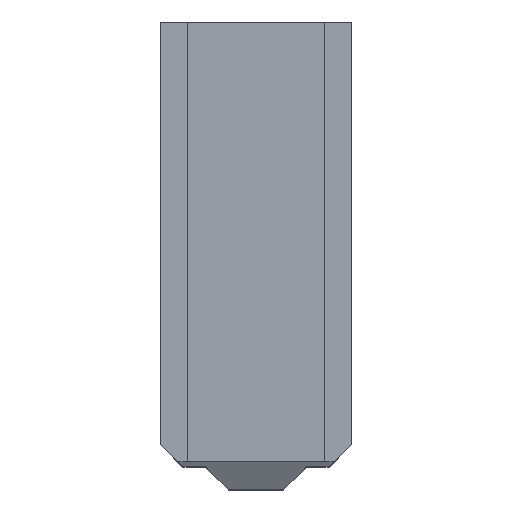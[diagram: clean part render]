
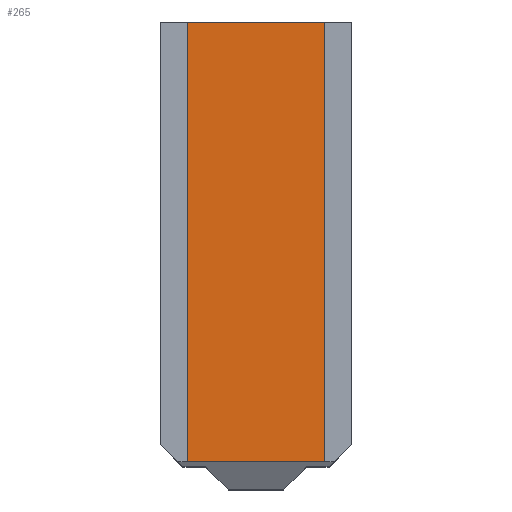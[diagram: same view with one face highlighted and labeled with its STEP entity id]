
A CAD part, top view. The second image highlights one B-rep face of the part: STEP entity #265.
In plain terms, the highlighted planar face has unit normal (0, 0, 1).
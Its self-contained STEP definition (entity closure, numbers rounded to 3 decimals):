
#164 = VERTEX_POINT ( 'NONE', #906 ) ;
#171 = VERTEX_POINT ( 'NONE', #882 ) ;
#204 = EDGE_LOOP ( 'NONE', ( #1276, #1154, #1141, #1271 ) ) ;
#229 = EDGE_CURVE ( 'NONE', #801, #812, #964, .T. ) ;
#265 = ADVANCED_FACE ( 'NONE', ( #513 ), #1112, .T. ) ;
#314 = EDGE_CURVE ( 'NONE', #171, #801, #1426, .T. ) ;
#315 = EDGE_CURVE ( 'NONE', #164, #171, #1428, .T. ) ;
#341 = EDGE_CURVE ( 'NONE', #812, #164, #1507, .T. ) ;
#444 = VECTOR ( 'NONE', #944, 1000. ) ;
#513 = FACE_OUTER_BOUND ( 'NONE', #204, .T. ) ;
#526 = AXIS2_PLACEMENT_3D ( 'NONE', #1099, #1109, #1105 ) ;
#599 = VECTOR ( 'NONE', #1427, 1000. ) ;
#608 = VECTOR ( 'NONE', #1468, 1000. ) ;
#624 = VECTOR ( 'NONE', #1511, 1000. ) ;
#801 = VERTEX_POINT ( 'NONE', #1573 ) ;
#812 = VERTEX_POINT ( 'NONE', #1560 ) ;
#882 = CARTESIAN_POINT ( 'NONE',  ( 15.128, -20.109, 114.412 ) ) ;
#906 = CARTESIAN_POINT ( 'NONE',  ( -15.113, -20.109, 114.412 ) ) ;
#943 = CARTESIAN_POINT ( 'NONE',  ( 0., 76.858, 114.412 ) ) ;
#944 = DIRECTION ( 'NONE',  ( -1., 0., 0. ) ) ;
#964 = LINE ( 'NONE', #943, #444 ) ;
#1099 = CARTESIAN_POINT ( 'NONE',  ( 0., 0., 114.412 ) ) ;
#1105 = DIRECTION ( 'NONE',  ( 1., 0., 0. ) ) ;
#1109 = DIRECTION ( 'NONE',  ( 0., 0., 1. ) ) ;
#1112 = PLANE ( 'NONE',  #526 ) ;
#1141 = ORIENTED_EDGE ( 'NONE', *, *, #229, .T. ) ;
#1154 = ORIENTED_EDGE ( 'NONE', *, *, #314, .T. ) ;
#1271 = ORIENTED_EDGE ( 'NONE', *, *, #341, .T. ) ;
#1276 = ORIENTED_EDGE ( 'NONE', *, *, #315, .T. ) ;
#1426 = LINE ( 'NONE', #1445, #599 ) ;
#1427 = DIRECTION ( 'NONE',  ( 0., 1., 0. ) ) ;
#1428 = LINE ( 'NONE', #1431, #608 ) ;
#1431 = CARTESIAN_POINT ( 'NONE',  ( 0., -20.109, 114.412 ) ) ;
#1445 = CARTESIAN_POINT ( 'NONE',  ( 15.128, 0., 114.412 ) ) ;
#1468 = DIRECTION ( 'NONE',  ( 1., 0., 0. ) ) ;
#1507 = LINE ( 'NONE', #1510, #624 ) ;
#1510 = CARTESIAN_POINT ( 'NONE',  ( -15.113, 0., 114.412 ) ) ;
#1511 = DIRECTION ( 'NONE',  ( 0., -1., 0. ) ) ;
#1560 = CARTESIAN_POINT ( 'NONE',  ( -15.112, 76.858, 114.412 ) ) ;
#1573 = CARTESIAN_POINT ( 'NONE',  ( 15.128, 76.858, 114.412 ) ) ;
